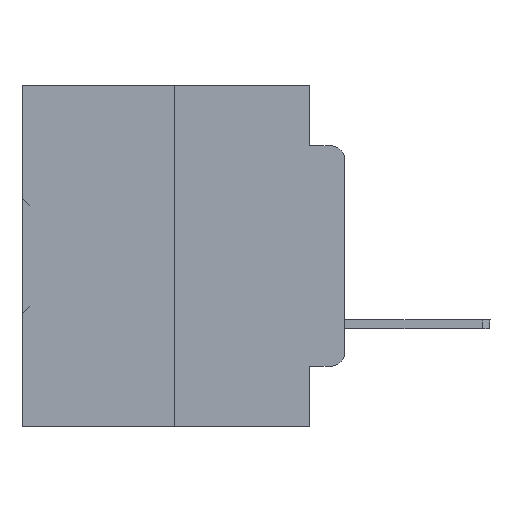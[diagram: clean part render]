
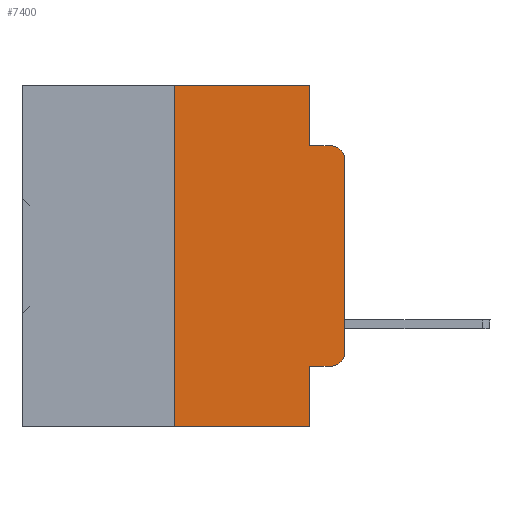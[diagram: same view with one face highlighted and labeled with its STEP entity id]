
A CAD part, left-side view. The second image highlights one B-rep face of the part: STEP entity #7400.
In plain terms, the highlighted planar face has unit normal (-1, 0, 0).
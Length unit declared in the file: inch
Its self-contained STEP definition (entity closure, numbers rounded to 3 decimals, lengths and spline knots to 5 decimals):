
#367 = CARTESIAN_POINT ( 'NONE',  ( 0., 0.02, -0.3915 ) ) ;
#1258 = VERTEX_POINT ( 'NONE', #23748 ) ;
#2425 = LINE ( 'NONE', #16527, #19121 ) ;
#2625 = LINE ( 'NONE', #14311, #31388 ) ;
#3494 = CARTESIAN_POINT ( 'NONE',  ( 0., 0., -0.3915 ) ) ;
#4004 = EDGE_CURVE ( 'NONE', #15023, #32125, #27690, .T. ) ;
#4597 = ORIENTED_EDGE ( 'NONE', *, *, #25062, .T. ) ;
#5258 = DIRECTION ( 'NONE',  ( 1., 0., 0. ) ) ;
#5627 = EDGE_CURVE ( 'NONE', #24504, #33828, #30332, .T. ) ;
#7289 = CARTESIAN_POINT ( 'NONE',  ( 0., 0.25, 0. ) ) ;
#7336 = ORIENTED_EDGE ( 'NONE', *, *, #27748, .T. ) ;
#7400 = ADVANCED_FACE ( 'NONE', ( #30664 ), #13414, .F. ) ;
#10062 = AXIS2_PLACEMENT_3D ( 'NONE', #18386, #12424, #12041 ) ;
#10881 = LINE ( 'NONE', #19254, #11625 ) ;
#11425 = VERTEX_POINT ( 'NONE', #23771 ) ;
#11624 = CARTESIAN_POINT ( 'NONE',  ( 0., 0.02, -0.0885 ) ) ;
#11625 = VECTOR ( 'NONE', #30565, 39.37008 ) ;
#12041 = DIRECTION ( 'NONE',  ( 0., 0., -1. ) ) ;
#12367 = AXIS2_PLACEMENT_3D ( 'NONE', #367, #26160, #29479 ) ;
#12424 = DIRECTION ( 'NONE',  ( -1., 0., 0. ) ) ;
#12441 = VERTEX_POINT ( 'NONE', #24488 ) ;
#13026 = DIRECTION ( 'NONE',  ( 0., -1., 0. ) ) ;
#13414 = PLANE ( 'NONE',  #28760 ) ;
#14304 = VERTEX_POINT ( 'NONE', #11624 ) ;
#14311 = CARTESIAN_POINT ( 'NONE',  ( 0., 0., 0. ) ) ;
#14365 = ORIENTED_EDGE ( 'NONE', *, *, #22982, .F. ) ;
#15023 = VERTEX_POINT ( 'NONE', #30676 ) ;
#16527 = CARTESIAN_POINT ( 'NONE',  ( 0., 0.051, 0. ) ) ;
#17219 = EDGE_CURVE ( 'NONE', #29344, #11425, #2625, .T. ) ;
#17292 = DIRECTION ( 'NONE',  ( 0., 0., 1. ) ) ;
#18007 = CARTESIAN_POINT ( 'NONE',  ( 0., 0.02, -0.4115 ) ) ;
#18173 = ORIENTED_EDGE ( 'NONE', *, *, #17219, .T. ) ;
#18386 = CARTESIAN_POINT ( 'NONE',  ( 0., 0.02, -0.1085 ) ) ;
#18811 = DIRECTION ( 'NONE',  ( 0., -1., 0. ) ) ;
#19121 = VECTOR ( 'NONE', #27641, 39.37008 ) ;
#19254 = CARTESIAN_POINT ( 'NONE',  ( 0., 0.051, -0.4115 ) ) ;
#20062 = EDGE_CURVE ( 'NONE', #33828, #12441, #2425, .T. ) ;
#21354 = CIRCLE ( 'NONE', #10062, 0.02 ) ;
#21415 = EDGE_CURVE ( 'NONE', #12441, #14304, #36251, .T. ) ;
#21578 = VECTOR ( 'NONE', #13026, 39.37008 ) ;
#21783 = CARTESIAN_POINT ( 'NONE',  ( 0., 0.051, 0. ) ) ;
#21886 = ORIENTED_EDGE ( 'NONE', *, *, #21415, .F. ) ;
#22830 = EDGE_LOOP ( 'NONE', ( #18173, #23094, #21886, #30743, #28254, #14365, #22858, #31831, #4597, #7336 ) ) ;
#22858 = ORIENTED_EDGE ( 'NONE', *, *, #4004, .T. ) ;
#22982 = EDGE_CURVE ( 'NONE', #15023, #24504, #26180, .T. ) ;
#23094 = ORIENTED_EDGE ( 'NONE', *, *, #30217, .T. ) ;
#23142 = VECTOR ( 'NONE', #35752, 39.37008 ) ;
#23748 = CARTESIAN_POINT ( 'NONE',  ( 0., 0.051, -0.4115 ) ) ;
#23771 = CARTESIAN_POINT ( 'NONE',  ( 0., 0., -0.1085 ) ) ;
#24488 = CARTESIAN_POINT ( 'NONE',  ( 0., 0.051, -0.0885 ) ) ;
#24504 = VERTEX_POINT ( 'NONE', #7289 ) ;
#24728 = CARTESIAN_POINT ( 'NONE',  ( 0., 0.473, 0. ) ) ;
#24912 = CARTESIAN_POINT ( 'NONE',  ( 0., 0.473, -0.5 ) ) ;
#24917 = DIRECTION ( 'NONE',  ( 0., 0., -1. ) ) ;
#25062 = EDGE_CURVE ( 'NONE', #1258, #28887, #10881, .T. ) ;
#25412 = CARTESIAN_POINT ( 'NONE',  ( 0., 0.051, 0. ) ) ;
#26160 = DIRECTION ( 'NONE',  ( -1., 0., 0. ) ) ;
#26180 = LINE ( 'NONE', #29500, #34068 ) ;
#26225 = VECTOR ( 'NONE', #18811, 39.37008 ) ;
#26611 = CIRCLE ( 'NONE', #12367, 0.02 ) ;
#27317 = CARTESIAN_POINT ( 'NONE',  ( 0., 0.051, -0.0885 ) ) ;
#27641 = DIRECTION ( 'NONE',  ( 0., 0., -1. ) ) ;
#27690 = LINE ( 'NONE', #24912, #26225 ) ;
#27748 = EDGE_CURVE ( 'NONE', #28887, #29344, #26611, .T. ) ;
#28254 = ORIENTED_EDGE ( 'NONE', *, *, #5627, .F. ) ;
#28760 = AXIS2_PLACEMENT_3D ( 'NONE', #24728, #5258, #24917 ) ;
#28887 = VERTEX_POINT ( 'NONE', #18007 ) ;
#29344 = VERTEX_POINT ( 'NONE', #3494 ) ;
#29442 = VECTOR ( 'NONE', #36288, 39.37008 ) ;
#29479 = DIRECTION ( 'NONE',  ( 0., 0., -1. ) ) ;
#29500 = CARTESIAN_POINT ( 'NONE',  ( 0., 0.25, 0. ) ) ;
#29941 = LINE ( 'NONE', #21783, #29442 ) ;
#30217 = EDGE_CURVE ( 'NONE', #11425, #14304, #21354, .T. ) ;
#30332 = LINE ( 'NONE', #32945, #23142 ) ;
#30565 = DIRECTION ( 'NONE',  ( 0., -1., 0. ) ) ;
#30664 = FACE_OUTER_BOUND ( 'NONE', #22830, .T. ) ;
#30676 = CARTESIAN_POINT ( 'NONE',  ( 0., 0.25, -0.5 ) ) ;
#30743 = ORIENTED_EDGE ( 'NONE', *, *, #20062, .F. ) ;
#31388 = VECTOR ( 'NONE', #17292, 39.37008 ) ;
#31831 = ORIENTED_EDGE ( 'NONE', *, *, #36357, .F. ) ;
#32125 = VERTEX_POINT ( 'NONE', #33725 ) ;
#32474 = DIRECTION ( 'NONE',  ( 0., 0., 1. ) ) ;
#32945 = CARTESIAN_POINT ( 'NONE',  ( 0., 0.473, 0. ) ) ;
#33725 = CARTESIAN_POINT ( 'NONE',  ( 0., 0.051, -0.5 ) ) ;
#33828 = VERTEX_POINT ( 'NONE', #25412 ) ;
#34068 = VECTOR ( 'NONE', #32474, 39.37008 ) ;
#35752 = DIRECTION ( 'NONE',  ( 0., -1., 0. ) ) ;
#36251 = LINE ( 'NONE', #27317, #21578 ) ;
#36288 = DIRECTION ( 'NONE',  ( 0., 0., -1. ) ) ;
#36357 = EDGE_CURVE ( 'NONE', #1258, #32125, #29941, .T. ) ;
